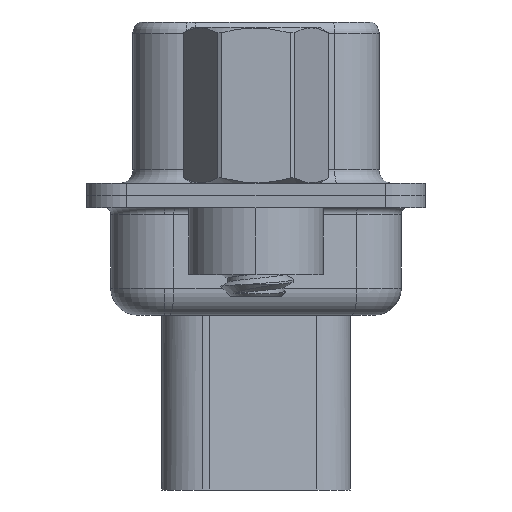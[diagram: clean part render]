
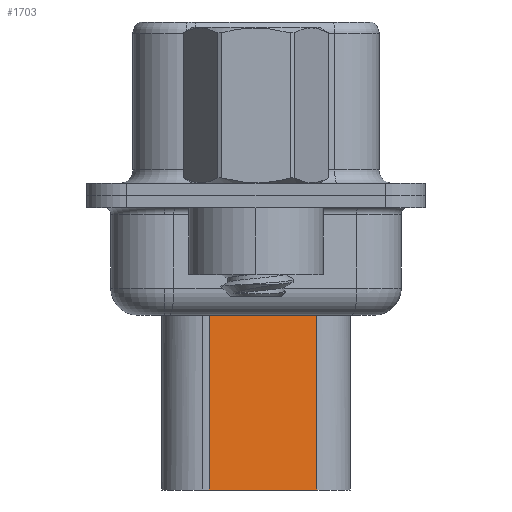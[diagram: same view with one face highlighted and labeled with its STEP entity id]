
A CAD part, left-side view. The second image highlights one B-rep face of the part: STEP entity #1703.
In plain terms, the highlighted planar face has unit normal (-0.985, -0.174, 0).
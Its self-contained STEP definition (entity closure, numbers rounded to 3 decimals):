
#1002 = VERTEX_POINT ( 'NONE', #9665 ) ;
#1196 = ORIENTED_EDGE ( 'NONE', *, *, #3790, .F. ) ;
#1252 = EDGE_LOOP ( 'NONE', ( #9079, #7112, #12194, #1196 ) ) ;
#1703 = ADVANCED_FACE ( 'NONE', ( #9029 ), #12604, .T. ) ;
#2852 = DIRECTION ( 'NONE',  ( 0., 0., -1. ) ) ;
#3309 = VECTOR ( 'NONE', #14238, 1000. ) ;
#3790 = EDGE_CURVE ( 'NONE', #5554, #12873, #15353, .T. ) ;
#3905 = DIRECTION ( 'NONE',  ( 0., 0., -1. ) ) ;
#4727 = CARTESIAN_POINT ( 'NONE',  ( 4.524, 1.74, -10.95 ) ) ;
#5090 = CARTESIAN_POINT ( 'NONE',  ( 4.524, 1.74, -10.95 ) ) ;
#5368 = LINE ( 'NONE', #15637, #12436 ) ;
#5495 = LINE ( 'NONE', #14727, #14389 ) ;
#5554 = VERTEX_POINT ( 'NONE', #12848 ) ;
#5749 = EDGE_CURVE ( 'NONE', #8707, #5554, #9377, .T. ) ;
#7112 = ORIENTED_EDGE ( 'NONE', *, *, #10636, .T. ) ;
#8329 = DIRECTION ( 'NONE',  ( -0.174, 0.985, 0. ) ) ;
#8707 = VERTEX_POINT ( 'NONE', #16254 ) ;
#8957 = EDGE_CURVE ( 'NONE', #1002, #12873, #5368, .T. ) ;
#9029 = FACE_OUTER_BOUND ( 'NONE', #1252, .T. ) ;
#9079 = ORIENTED_EDGE ( 'NONE', *, *, #5749, .F. ) ;
#9377 = LINE ( 'NONE', #14575, #11300 ) ;
#9665 = CARTESIAN_POINT ( 'NONE',  ( 4.524, 1.74, -3.975 ) ) ;
#10224 = CARTESIAN_POINT ( 'NONE',  ( 4.524, 1.74, -3.1 ) ) ;
#10636 = EDGE_CURVE ( 'NONE', #8707, #1002, #5495, .T. ) ;
#11300 = VECTOR ( 'NONE', #2852, 1000. ) ;
#12194 = ORIENTED_EDGE ( 'NONE', *, *, #8957, .T. ) ;
#12436 = VECTOR ( 'NONE', #3905, 1000. ) ;
#12604 = PLANE ( 'NONE',  #14029 ) ;
#12848 = CARTESIAN_POINT ( 'NONE',  ( 5.229, -2.26, -10.95 ) ) ;
#12873 = VERTEX_POINT ( 'NONE', #4727 ) ;
#14029 = AXIS2_PLACEMENT_3D ( 'NONE', #10224, #15433, #14227 ) ;
#14227 = DIRECTION ( 'NONE',  ( 0.174, -0.985, 0. ) ) ;
#14238 = DIRECTION ( 'NONE',  ( -0.174, 0.985, 0. ) ) ;
#14389 = VECTOR ( 'NONE', #8329, 1000. ) ;
#14575 = CARTESIAN_POINT ( 'NONE',  ( 5.229, -2.26, -3.1 ) ) ;
#14727 = CARTESIAN_POINT ( 'NONE',  ( 4.353, 2.709, -3.975 ) ) ;
#15353 = LINE ( 'NONE', #5090, #3309 ) ;
#15433 = DIRECTION ( 'NONE',  ( -0.985, -0.174, 0. ) ) ;
#15637 = CARTESIAN_POINT ( 'NONE',  ( 4.524, 1.74, -3.1 ) ) ;
#16254 = CARTESIAN_POINT ( 'NONE',  ( 5.229, -2.26, -3.975 ) ) ;
